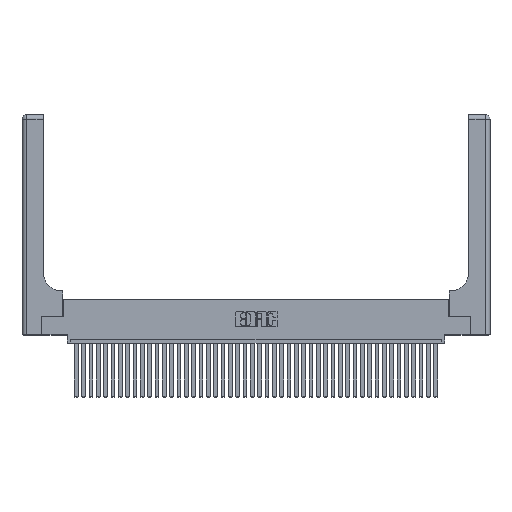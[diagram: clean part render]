
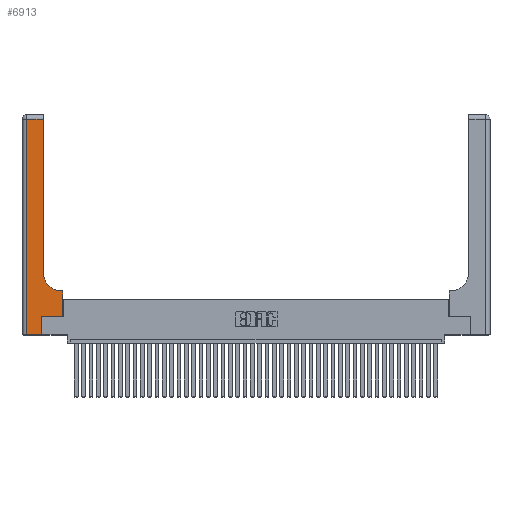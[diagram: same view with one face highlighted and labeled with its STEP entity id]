
A CAD part, top view. The second image highlights one B-rep face of the part: STEP entity #6913.
In plain terms, the highlighted planar face has unit normal (0, 0, 1).
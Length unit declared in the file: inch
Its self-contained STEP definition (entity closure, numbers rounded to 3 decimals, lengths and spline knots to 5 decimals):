
#281 = LINE ( 'NONE', #8631, #25076 ) ;
#1281 = CARTESIAN_POINT ( 'NONE',  ( 0.06, 2.94, 0.37 ) ) ;
#1597 = EDGE_CURVE ( 'NONE', #31299, #19305, #40565, .T. ) ;
#2691 = VECTOR ( 'NONE', #39591, 39.37008 ) ;
#3039 = CARTESIAN_POINT ( 'NONE',  ( 0.269, 0.25, 0.37 ) ) ;
#3147 = ORIENTED_EDGE ( 'NONE', *, *, #11052, .T. ) ;
#3855 = VECTOR ( 'NONE', #19888, 39.37008 ) ;
#4276 = LINE ( 'NONE', #32498, #7847 ) ;
#4590 = VERTEX_POINT ( 'NONE', #21578 ) ;
#4798 = CIRCLE ( 'NONE', #25052, 0.25 ) ;
#5764 = PLANE ( 'NONE',  #40598 ) ;
#6312 = CARTESIAN_POINT ( 'NONE',  ( 0.2915, 0.85, 0.37 ) ) ;
#6545 = VERTEX_POINT ( 'NONE', #25871 ) ;
#6898 = ORIENTED_EDGE ( 'NONE', *, *, #17981, .T. ) ;
#6904 = LINE ( 'NONE', #3039, #3855 ) ;
#6913 = ADVANCED_FACE ( 'NONE', ( #35227 ), #5764, .F. ) ;
#7072 = DIRECTION ( 'NONE',  ( 0., 1., 0. ) ) ;
#7196 = LINE ( 'NONE', #21172, #31910 ) ;
#7652 = CARTESIAN_POINT ( 'NONE',  ( 0.5415, 0.6, 0.37 ) ) ;
#7847 = VECTOR ( 'NONE', #26916, 39.37008 ) ;
#8299 = EDGE_CURVE ( 'NONE', #31952, #38453, #6904, .T. ) ;
#8631 = CARTESIAN_POINT ( 'NONE',  ( 0.06, 3., 0.37 ) ) ;
#9047 = CARTESIAN_POINT ( 'NONE',  ( 0., 3., 0.37 ) ) ;
#9359 = CARTESIAN_POINT ( 'NONE',  ( 0., 2.94, 0.37 ) ) ;
#10414 = CARTESIAN_POINT ( 'NONE',  ( 0.269, 0.25, 0.37 ) ) ;
#11052 = EDGE_CURVE ( 'NONE', #4590, #31952, #31392, .T. ) ;
#11420 = ORIENTED_EDGE ( 'NONE', *, *, #34982, .T. ) ;
#14370 = ORIENTED_EDGE ( 'NONE', *, *, #1597, .T. ) ;
#15028 = DIRECTION ( 'NONE',  ( 1., 0., 0. ) ) ;
#17907 = DIRECTION ( 'NONE',  ( 1., 0., 0. ) ) ;
#17981 = EDGE_CURVE ( 'NONE', #38453, #31299, #4276, .T. ) ;
#18688 = EDGE_CURVE ( 'NONE', #19619, #4590, #7196, .T. ) ;
#19305 = VERTEX_POINT ( 'NONE', #7652 ) ;
#19619 = VERTEX_POINT ( 'NONE', #40488 ) ;
#19888 = DIRECTION ( 'NONE',  ( 1., 0., 0. ) ) ;
#19905 = VECTOR ( 'NONE', #41393, 39.37008 ) ;
#20354 = VERTEX_POINT ( 'NONE', #1281 ) ;
#20999 = ORIENTED_EDGE ( 'NONE', *, *, #18688, .T. ) ;
#21172 = CARTESIAN_POINT ( 'NONE',  ( 0., 0., 0.37 ) ) ;
#21578 = CARTESIAN_POINT ( 'NONE',  ( 0.269, 0., 0.37 ) ) ;
#22775 = EDGE_CURVE ( 'NONE', #20354, #19619, #281, .T. ) ;
#22878 = VECTOR ( 'NONE', #32078, 39.37008 ) ;
#23102 = CARTESIAN_POINT ( 'NONE',  ( 0.5585, 0.6, 0.37 ) ) ;
#23827 = LINE ( 'NONE', #39285, #30886 ) ;
#25050 = LINE ( 'NONE', #9359, #19905 ) ;
#25052 = AXIS2_PLACEMENT_3D ( 'NONE', #40484, #34239, #15028 ) ;
#25076 = VECTOR ( 'NONE', #37285, 39.37008 ) ;
#25159 = CARTESIAN_POINT ( 'NONE',  ( 0.5585, 0.25, 0.37 ) ) ;
#25871 = CARTESIAN_POINT ( 'NONE',  ( 0.2915, 2.94, 0.37 ) ) ;
#26300 = ORIENTED_EDGE ( 'NONE', *, *, #29192, .T. ) ;
#26916 = DIRECTION ( 'NONE',  ( 0., 1., 0. ) ) ;
#27123 = CARTESIAN_POINT ( 'NONE',  ( 0.269, 0., 0.37 ) ) ;
#28872 = CARTESIAN_POINT ( 'NONE',  ( 0.2915, 0.6, 0.37 ) ) ;
#29192 = EDGE_CURVE ( 'NONE', #6545, #20354, #25050, .T. ) ;
#30886 = VECTOR ( 'NONE', #7072, 39.37008 ) ;
#31299 = VERTEX_POINT ( 'NONE', #23102 ) ;
#31392 = LINE ( 'NONE', #27123, #2691 ) ;
#31910 = VECTOR ( 'NONE', #17907, 39.37008 ) ;
#31952 = VERTEX_POINT ( 'NONE', #10414 ) ;
#32032 = DIRECTION ( 'NONE',  ( -1., 0., 0. ) ) ;
#32078 = DIRECTION ( 'NONE',  ( -1., 0., 0. ) ) ;
#32498 = CARTESIAN_POINT ( 'NONE',  ( 0.5585, 0.25, 0.37 ) ) ;
#33479 = ORIENTED_EDGE ( 'NONE', *, *, #36878, .T. ) ;
#34239 = DIRECTION ( 'NONE',  ( 0., 0., -1. ) ) ;
#34572 = VERTEX_POINT ( 'NONE', #6312 ) ;
#34982 = EDGE_CURVE ( 'NONE', #19305, #34572, #4798, .T. ) ;
#35227 = FACE_OUTER_BOUND ( 'NONE', #35236, .T. ) ;
#35236 = EDGE_LOOP ( 'NONE', ( #33479, #26300, #36658, #20999, #3147, #36034, #6898, #14370, #11420 ) ) ;
#36034 = ORIENTED_EDGE ( 'NONE', *, *, #8299, .T. ) ;
#36658 = ORIENTED_EDGE ( 'NONE', *, *, #22775, .T. ) ;
#36878 = EDGE_CURVE ( 'NONE', #34572, #6545, #23827, .T. ) ;
#37285 = DIRECTION ( 'NONE',  ( 0., -1., 0. ) ) ;
#37984 = DIRECTION ( 'NONE',  ( 0., 0., -1. ) ) ;
#38453 = VERTEX_POINT ( 'NONE', #25159 ) ;
#39285 = CARTESIAN_POINT ( 'NONE',  ( 0.2915, 3., 0.37 ) ) ;
#39591 = DIRECTION ( 'NONE',  ( 0., 1., 0. ) ) ;
#40484 = CARTESIAN_POINT ( 'NONE',  ( 0.5415, 0.85, 0.37 ) ) ;
#40488 = CARTESIAN_POINT ( 'NONE',  ( 0.06, 0., 0.37 ) ) ;
#40565 = LINE ( 'NONE', #28872, #22878 ) ;
#40598 = AXIS2_PLACEMENT_3D ( 'NONE', #9047, #37984, #32032 ) ;
#41393 = DIRECTION ( 'NONE',  ( -1., 0., 0. ) ) ;
